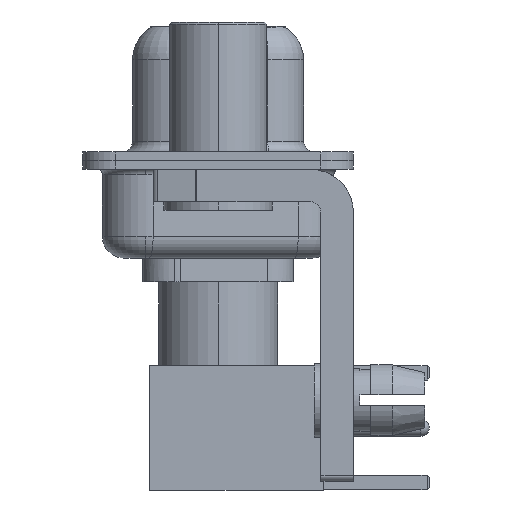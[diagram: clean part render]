
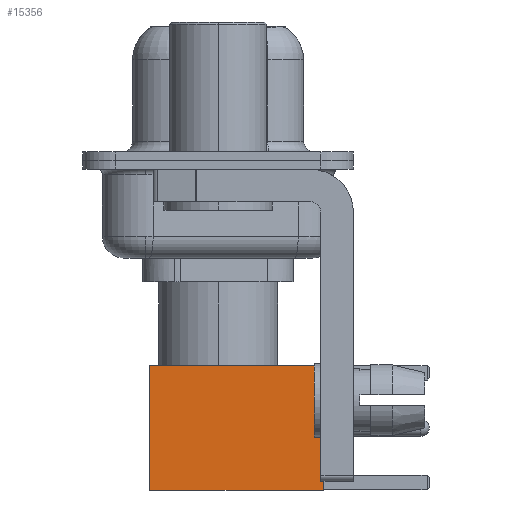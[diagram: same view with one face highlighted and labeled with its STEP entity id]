
A CAD part, left-side view. The second image highlights one B-rep face of the part: STEP entity #15356.
In plain terms, the highlighted face is planar.
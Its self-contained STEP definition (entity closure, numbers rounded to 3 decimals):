
#76 = AXIS2_PLACEMENT_3D ( 'NONE', #19356, #5371, #12061 ) ;
#882 = VERTEX_POINT ( 'NONE', #7753 ) ;
#938 = ORIENTED_EDGE ( 'NONE', *, *, #22401, .F. ) ;
#3415 = EDGE_CURVE ( 'NONE', #11257, #21970, #20430, .T. ) ;
#3525 = DIRECTION ( 'NONE',  ( -1., 0., 0. ) ) ;
#3639 = LINE ( 'NONE', #14197, #20787 ) ;
#3766 = FACE_OUTER_BOUND ( 'NONE', #4673, .T. ) ;
#3884 = DIRECTION ( 'NONE',  ( 0., 0., -1. ) ) ;
#4589 = CARTESIAN_POINT ( 'NONE',  ( 2.875, 2.875, 8. ) ) ;
#4673 = EDGE_LOOP ( 'NONE', ( #5941, #7343, #10109, #938 ) ) ;
#5371 = DIRECTION ( 'NONE',  ( 0., 1., 0. ) ) ;
#5442 = VERTEX_POINT ( 'NONE', #4589 ) ;
#5941 = ORIENTED_EDGE ( 'NONE', *, *, #16988, .T. ) ;
#7343 = ORIENTED_EDGE ( 'NONE', *, *, #3415, .T. ) ;
#7753 = CARTESIAN_POINT ( 'NONE',  ( -2.875, 2.875, 8. ) ) ;
#8369 = DIRECTION ( 'NONE',  ( -1., 0., 0. ) ) ;
#9118 = DIRECTION ( 'NONE',  ( 0., 0., -1. ) ) ;
#9225 = CARTESIAN_POINT ( 'NONE',  ( 2.875, 2.875, 0. ) ) ;
#10109 = ORIENTED_EDGE ( 'NONE', *, *, #15543, .F. ) ;
#10413 = CARTESIAN_POINT ( 'NONE',  ( 0., 2.875, 0. ) ) ;
#11009 = CARTESIAN_POINT ( 'NONE',  ( 2.875, 2.875, 0. ) ) ;
#11257 = VERTEX_POINT ( 'NONE', #11009 ) ;
#12061 = DIRECTION ( 'NONE',  ( 0., 0., 1. ) ) ;
#12172 = CARTESIAN_POINT ( 'NONE',  ( -2.875, 2.875, 0. ) ) ;
#12399 = LINE ( 'NONE', #19470, #22290 ) ;
#12438 = VECTOR ( 'NONE', #9118, 1000. ) ;
#13878 = PLANE ( 'NONE',  #76 ) ;
#14197 = CARTESIAN_POINT ( 'NONE',  ( 0., 2.875, 8. ) ) ;
#15356 = ADVANCED_FACE ( 'NONE', ( #3766 ), #13878, .T. ) ;
#15543 = EDGE_CURVE ( 'NONE', #882, #21970, #12399, .T. ) ;
#16988 = EDGE_CURVE ( 'NONE', #5442, #11257, #21087, .T. ) ;
#19356 = CARTESIAN_POINT ( 'NONE',  ( 2.875, 2.875, 0. ) ) ;
#19470 = CARTESIAN_POINT ( 'NONE',  ( -2.875, 2.875, 0. ) ) ;
#20430 = LINE ( 'NONE', #10413, #22031 ) ;
#20787 = VECTOR ( 'NONE', #3525, 1000. ) ;
#21087 = LINE ( 'NONE', #9225, #12438 ) ;
#21970 = VERTEX_POINT ( 'NONE', #12172 ) ;
#22031 = VECTOR ( 'NONE', #8369, 1000. ) ;
#22290 = VECTOR ( 'NONE', #3884, 1000. ) ;
#22401 = EDGE_CURVE ( 'NONE', #5442, #882, #3639, .T. ) ;
